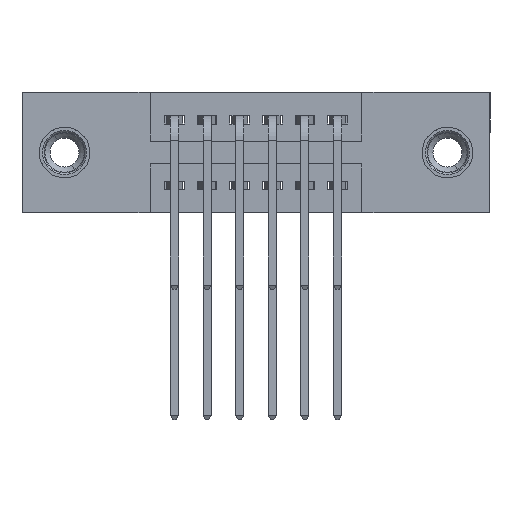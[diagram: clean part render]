
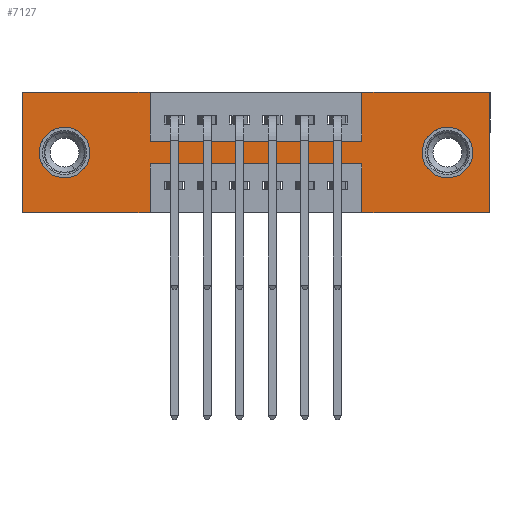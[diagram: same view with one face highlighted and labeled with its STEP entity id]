
A CAD part, front view. The second image highlights one B-rep face of the part: STEP entity #7127.
In plain terms, the highlighted planar face has unit normal (0, -1, 0).
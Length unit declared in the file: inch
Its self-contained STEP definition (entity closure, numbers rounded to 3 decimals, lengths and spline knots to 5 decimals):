
#6 = AXIS2_PLACEMENT_3D ( 'NONE', #14995, #13972, #1743 ) ;
#126 = AXIS2_PLACEMENT_3D ( 'NONE', #11579, #10801, #5903 ) ;
#598 = EDGE_CURVE ( 'NONE', #1256, #5711, #13879, .T. ) ;
#843 = DIRECTION ( 'NONE',  ( 0., 0., -1. ) ) ;
#880 = DIRECTION ( 'NONE',  ( 0., 0., 1. ) ) ;
#967 = CARTESIAN_POINT ( 'NONE',  ( 0., 0., 0. ) ) ;
#1009 = LINE ( 'NONE', #8261, #14521 ) ;
#1256 = VERTEX_POINT ( 'NONE', #3262 ) ;
#1290 = CARTESIAN_POINT ( 'NONE',  ( 0.3925, 0., -0.37 ) ) ;
#1396 = AXIS2_PLACEMENT_3D ( 'NONE', #14464, #10767, #880 ) ;
#1428 = PLANE ( 'NONE',  #6 ) ;
#1531 = CARTESIAN_POINT ( 'NONE',  ( 1.0425, 0., -0.37 ) ) ;
#1629 = LINE ( 'NONE', #6940, #6856 ) ;
#1743 = DIRECTION ( 'NONE',  ( 0., 0., -1. ) ) ;
#1851 = CIRCLE ( 'NONE', #2632, 0.078 ) ;
#2178 = ORIENTED_EDGE ( 'NONE', *, *, #11085, .T. ) ;
#2195 = VERTEX_POINT ( 'NONE', #3070 ) ;
#2198 = DIRECTION ( 'NONE',  ( 1., 0., 0. ) ) ;
#2218 = EDGE_CURVE ( 'NONE', #11496, #13370, #14055, .T. ) ;
#2260 = ORIENTED_EDGE ( 'NONE', *, *, #9318, .T. ) ;
#2589 = ORIENTED_EDGE ( 'NONE', *, *, #2218, .F. ) ;
#2632 = AXIS2_PLACEMENT_3D ( 'NONE', #14291, #5683, #5586 ) ;
#2643 = ORIENTED_EDGE ( 'NONE', *, *, #3122, .F. ) ;
#2666 = CARTESIAN_POINT ( 'NONE',  ( 0., 0., -0.37 ) ) ;
#2977 = AXIS2_PLACEMENT_3D ( 'NONE', #12365, #5011, #6240 ) ;
#3017 = EDGE_LOOP ( 'NONE', ( #7092, #15765, #13121, #8945, #4102, #5969, #7122, #4058, #2589, #6336, #9490, #2643 ) ) ;
#3070 = CARTESIAN_POINT ( 'NONE',  ( 1.435, 0., 0. ) ) ;
#3122 = EDGE_CURVE ( 'NONE', #5418, #4362, #14226, .T. ) ;
#3146 = EDGE_CURVE ( 'NONE', #5393, #5418, #9946, .T. ) ;
#3228 = CARTESIAN_POINT ( 'NONE',  ( 0.3925, 0., 0. ) ) ;
#3262 = CARTESIAN_POINT ( 'NONE',  ( 1.435, 0., -0.37 ) ) ;
#3352 = FACE_BOUND ( 'NONE', #14656, .T. ) ;
#3395 = EDGE_CURVE ( 'NONE', #4752, #5035, #13623, .T. ) ;
#3417 = DIRECTION ( 'NONE',  ( 0., 0., -1. ) ) ;
#3527 = DIRECTION ( 'NONE',  ( 0., 0., 1. ) ) ;
#3774 = LINE ( 'NONE', #14483, #12414 ) ;
#4058 = ORIENTED_EDGE ( 'NONE', *, *, #11158, .F. ) ;
#4102 = ORIENTED_EDGE ( 'NONE', *, *, #11723, .F. ) ;
#4362 = VERTEX_POINT ( 'NONE', #2666 ) ;
#4472 = DIRECTION ( 'NONE',  ( 1., 0., 0. ) ) ;
#4566 = DIRECTION ( 'NONE',  ( -1., 0., 0. ) ) ;
#4636 = CIRCLE ( 'NONE', #126, 0.078 ) ;
#4746 = LINE ( 'NONE', #12827, #10883 ) ;
#4752 = VERTEX_POINT ( 'NONE', #7671 ) ;
#5011 = DIRECTION ( 'NONE',  ( 0., 1., 0. ) ) ;
#5021 = VECTOR ( 'NONE', #3527, 39.37008 ) ;
#5035 = VERTEX_POINT ( 'NONE', #7675 ) ;
#5312 = VECTOR ( 'NONE', #3417, 39.37008 ) ;
#5393 = VERTEX_POINT ( 'NONE', #15991 ) ;
#5418 = VERTEX_POINT ( 'NONE', #1290 ) ;
#5586 = DIRECTION ( 'NONE',  ( 0., 0., -1. ) ) ;
#5639 = DIRECTION ( 'NONE',  ( 1., 0., 0. ) ) ;
#5683 = DIRECTION ( 'NONE',  ( 0., 1., 0. ) ) ;
#5709 = CARTESIAN_POINT ( 'NONE',  ( 1.305, 0., -0.263 ) ) ;
#5711 = VERTEX_POINT ( 'NONE', #1531 ) ;
#5799 = CARTESIAN_POINT ( 'NONE',  ( 0., 0., -0.37 ) ) ;
#5903 = DIRECTION ( 'NONE',  ( 0., 0., -1. ) ) ;
#5969 = ORIENTED_EDGE ( 'NONE', *, *, #10777, .F. ) ;
#6066 = CARTESIAN_POINT ( 'NONE',  ( 1.0425, 0., -0.15 ) ) ;
#6240 = DIRECTION ( 'NONE',  ( 0., 0., 1. ) ) ;
#6336 = ORIENTED_EDGE ( 'NONE', *, *, #12783, .F. ) ;
#6369 = DIRECTION ( 'NONE',  ( 0., 0., 1. ) ) ;
#6481 = CARTESIAN_POINT ( 'NONE',  ( 0., 0., 0. ) ) ;
#6507 = VERTEX_POINT ( 'NONE', #967 ) ;
#6856 = VECTOR ( 'NONE', #4566, 39.37008 ) ;
#6940 = CARTESIAN_POINT ( 'NONE',  ( 0.3925, 0., -0.22 ) ) ;
#7092 = ORIENTED_EDGE ( 'NONE', *, *, #3146, .F. ) ;
#7122 = ORIENTED_EDGE ( 'NONE', *, *, #9925, .F. ) ;
#7127 = ADVANCED_FACE ( 'NONE', ( #3352, #8203, #13559 ), #1428, .T. ) ;
#7671 = CARTESIAN_POINT ( 'NONE',  ( 0.13, 0., -0.263 ) ) ;
#7675 = CARTESIAN_POINT ( 'NONE',  ( 0.13, 0., -0.107 ) ) ;
#8001 = VERTEX_POINT ( 'NONE', #15216 ) ;
#8203 = FACE_BOUND ( 'NONE', #10016, .T. ) ;
#8261 = CARTESIAN_POINT ( 'NONE',  ( 0., 0., 0. ) ) ;
#8284 = CARTESIAN_POINT ( 'NONE',  ( 1.0425, 0., -0.22 ) ) ;
#8480 = VECTOR ( 'NONE', #14147, 39.37008 ) ;
#8495 = VECTOR ( 'NONE', #15670, 39.37008 ) ;
#8631 = ORIENTED_EDGE ( 'NONE', *, *, #3395, .T. ) ;
#8688 = LINE ( 'NONE', #15827, #5021 ) ;
#8689 = VERTEX_POINT ( 'NONE', #12042 ) ;
#8945 = ORIENTED_EDGE ( 'NONE', *, *, #598, .F. ) ;
#9142 = CARTESIAN_POINT ( 'NONE',  ( 0.3925, 0., -0.15 ) ) ;
#9204 = VECTOR ( 'NONE', #843, 39.37008 ) ;
#9318 = EDGE_CURVE ( 'NONE', #8001, #11668, #4636, .T. ) ;
#9490 = ORIENTED_EDGE ( 'NONE', *, *, #13740, .F. ) ;
#9757 = CARTESIAN_POINT ( 'NONE',  ( 1.435, 0., 0. ) ) ;
#9925 = EDGE_CURVE ( 'NONE', #13004, #8689, #15017, .T. ) ;
#9946 = LINE ( 'NONE', #11779, #9204 ) ;
#10016 = EDGE_LOOP ( 'NONE', ( #10190, #8631 ) ) ;
#10190 = ORIENTED_EDGE ( 'NONE', *, *, #10585, .T. ) ;
#10585 = EDGE_CURVE ( 'NONE', #5035, #4752, #11885, .T. ) ;
#10663 = LINE ( 'NONE', #9757, #5312 ) ;
#10767 = DIRECTION ( 'NONE',  ( 0., 1., 0. ) ) ;
#10769 = CARTESIAN_POINT ( 'NONE',  ( 0., 0., -0.37 ) ) ;
#10777 = EDGE_CURVE ( 'NONE', #8689, #2195, #3774, .T. ) ;
#10801 = DIRECTION ( 'NONE',  ( 0., 1., 0. ) ) ;
#10883 = VECTOR ( 'NONE', #5639, 39.37008 ) ;
#11085 = EDGE_CURVE ( 'NONE', #11668, #8001, #1851, .T. ) ;
#11158 = EDGE_CURVE ( 'NONE', #13370, #13004, #4746, .T. ) ;
#11217 = VERTEX_POINT ( 'NONE', #8284 ) ;
#11496 = VERTEX_POINT ( 'NONE', #11800 ) ;
#11579 = CARTESIAN_POINT ( 'NONE',  ( 1.305, 0., -0.185 ) ) ;
#11668 = VERTEX_POINT ( 'NONE', #5709 ) ;
#11676 = EDGE_CURVE ( 'NONE', #11217, #5393, #1629, .T. ) ;
#11723 = EDGE_CURVE ( 'NONE', #2195, #1256, #10663, .T. ) ;
#11779 = CARTESIAN_POINT ( 'NONE',  ( 0.3925, 0., -0.37 ) ) ;
#11800 = CARTESIAN_POINT ( 'NONE',  ( 0.3925, 0., 0. ) ) ;
#11885 = CIRCLE ( 'NONE', #1396, 0.078 ) ;
#12042 = CARTESIAN_POINT ( 'NONE',  ( 1.0425, 0., 0. ) ) ;
#12365 = CARTESIAN_POINT ( 'NONE',  ( 0.13, 0., -0.185 ) ) ;
#12414 = VECTOR ( 'NONE', #2198, 39.37008 ) ;
#12527 = VECTOR ( 'NONE', #6369, 39.37008 ) ;
#12783 = EDGE_CURVE ( 'NONE', #6507, #11496, #1009, .T. ) ;
#12827 = CARTESIAN_POINT ( 'NONE',  ( 0.3925, 0., -0.15 ) ) ;
#12879 = VECTOR ( 'NONE', #15683, 39.37008 ) ;
#12940 = LINE ( 'NONE', #6481, #12527 ) ;
#13004 = VERTEX_POINT ( 'NONE', #6066 ) ;
#13059 = DIRECTION ( 'NONE',  ( -1., 0., 0. ) ) ;
#13121 = ORIENTED_EDGE ( 'NONE', *, *, #14998, .F. ) ;
#13370 = VERTEX_POINT ( 'NONE', #9142 ) ;
#13559 = FACE_OUTER_BOUND ( 'NONE', #3017, .T. ) ;
#13623 = CIRCLE ( 'NONE', #2977, 0.078 ) ;
#13740 = EDGE_CURVE ( 'NONE', #4362, #6507, #12940, .T. ) ;
#13832 = VECTOR ( 'NONE', #13059, 39.37008 ) ;
#13879 = LINE ( 'NONE', #10769, #8495 ) ;
#13972 = DIRECTION ( 'NONE',  ( 0., -1., 0. ) ) ;
#14055 = LINE ( 'NONE', #3228, #12879 ) ;
#14147 = DIRECTION ( 'NONE',  ( 0., 0., 1. ) ) ;
#14226 = LINE ( 'NONE', #5799, #13832 ) ;
#14291 = CARTESIAN_POINT ( 'NONE',  ( 1.305, 0., -0.185 ) ) ;
#14311 = CARTESIAN_POINT ( 'NONE',  ( 1.0425, 0., 0. ) ) ;
#14464 = CARTESIAN_POINT ( 'NONE',  ( 0.13, 0., -0.185 ) ) ;
#14483 = CARTESIAN_POINT ( 'NONE',  ( 0., 0., 0. ) ) ;
#14521 = VECTOR ( 'NONE', #4472, 39.37008 ) ;
#14656 = EDGE_LOOP ( 'NONE', ( #2260, #2178 ) ) ;
#14995 = CARTESIAN_POINT ( 'NONE',  ( 0., 0., -0.37 ) ) ;
#14998 = EDGE_CURVE ( 'NONE', #5711, #11217, #8688, .T. ) ;
#15017 = LINE ( 'NONE', #14311, #8480 ) ;
#15216 = CARTESIAN_POINT ( 'NONE',  ( 1.305, 0., -0.107 ) ) ;
#15670 = DIRECTION ( 'NONE',  ( -1., 0., 0. ) ) ;
#15683 = DIRECTION ( 'NONE',  ( 0., 0., -1. ) ) ;
#15765 = ORIENTED_EDGE ( 'NONE', *, *, #11676, .F. ) ;
#15827 = CARTESIAN_POINT ( 'NONE',  ( 1.0425, 0., -0.37 ) ) ;
#15991 = CARTESIAN_POINT ( 'NONE',  ( 0.3925, 0., -0.22 ) ) ;
